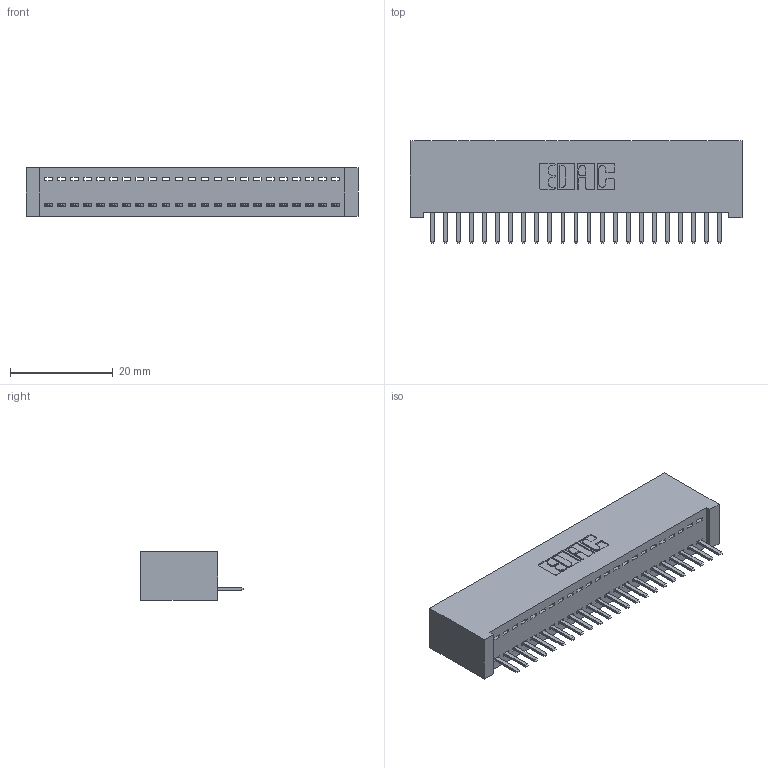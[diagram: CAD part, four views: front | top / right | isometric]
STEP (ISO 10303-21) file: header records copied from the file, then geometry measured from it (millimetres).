
FILE_DESCRIPTION (( 'STEP AP203' ), '1' );
FILE_NAME ('392-023-520-101.STEP', '2018-08-15T13:16:42', ( '' ), ( '' ), 'SwSTEP 2.0', 'SolidWorks 2016', '' );
FILE_SCHEMA (( 'CONFIG_CONTROL_DESIGN' ));
Length unit declared in the file: inch
Products named in the file (3): 342 Part_Lugless; 345-292-001_345-293-120; 392-023-520-101
Assembly tree (24 placements, depth 2):
  392-023-520-101
    342 Part_Lugless
    345-292-001_345-293-120  x23
Bounding box: 64.67 x 20.02 x 9.4 mm (x, y, z)
Volume: 5943 mm3; surface area: 8483.9 mm2
Topology: 24 solids, 24 shells, 1528 faces, 4507 edges, 2942 vertices
Faces by surface type: plane 1074, cylinder 454
Entity records: 16223 total; most frequent: CARTESIAN_POINT 2819, ORIENTED_EDGE 2766, DIRECTION 2397, EDGE_CURVE 1383, VECTOR 1259, LINE 1259, VERTEX_POINT 918, AXIS2_PLACEMENT_3D 569
